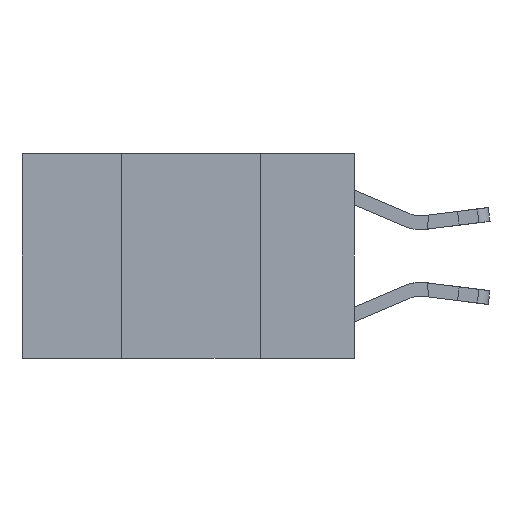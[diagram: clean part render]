
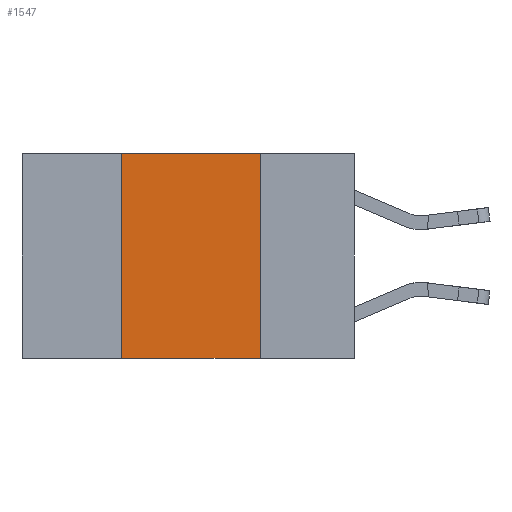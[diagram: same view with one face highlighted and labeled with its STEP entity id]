
A CAD part, left-side view. The second image highlights one B-rep face of the part: STEP entity #1547.
In plain terms, the highlighted planar face has unit normal (-1, 0, 0).
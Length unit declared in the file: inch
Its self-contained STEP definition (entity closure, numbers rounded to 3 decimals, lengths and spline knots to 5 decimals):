
#706 = VECTOR ( 'NONE', #12250, 39.37008 ) ;
#799 = LINE ( 'NONE', #14704, #10522 ) ;
#994 = DIRECTION ( 'NONE',  ( 0., -1., 0. ) ) ;
#1257 = VERTEX_POINT ( 'NONE', #6900 ) ;
#1547 = ADVANCED_FACE ( 'NONE', ( #10801 ), #2718, .F. ) ;
#2061 = VECTOR ( 'NONE', #11833, 39.37008 ) ;
#2718 = PLANE ( 'NONE',  #9936 ) ;
#3215 = ORIENTED_EDGE ( 'NONE', *, *, #4016, .F. ) ;
#3453 = CARTESIAN_POINT ( 'NONE',  ( 0., 0.6, -0.37 ) ) ;
#3618 = VERTEX_POINT ( 'NONE', #4906 ) ;
#3799 = ORIENTED_EDGE ( 'NONE', *, *, #6471, .F. ) ;
#4015 = LINE ( 'NONE', #11058, #706 ) ;
#4016 = EDGE_CURVE ( 'NONE', #3618, #1257, #8946, .T. ) ;
#4339 = EDGE_LOOP ( 'NONE', ( #10075, #3215, #3799, #9729 ) ) ;
#4906 = CARTESIAN_POINT ( 'NONE',  ( 0., 0.42, 0. ) ) ;
#5204 = DIRECTION ( 'NONE',  ( 0., 0., -1. ) ) ;
#5655 = EDGE_CURVE ( 'NONE', #6476, #13946, #10934, .T. ) ;
#5852 = CARTESIAN_POINT ( 'NONE',  ( 0., 0.6, 0. ) ) ;
#6471 = EDGE_CURVE ( 'NONE', #6476, #3618, #799, .T. ) ;
#6476 = VERTEX_POINT ( 'NONE', #13464 ) ;
#6900 = CARTESIAN_POINT ( 'NONE',  ( 0., 0.17, 0. ) ) ;
#7545 = DIRECTION ( 'NONE',  ( 0., 0., 1. ) ) ;
#7910 = CARTESIAN_POINT ( 'NONE',  ( 0., 0.17, -0.37 ) ) ;
#8946 = LINE ( 'NONE', #5852, #2061 ) ;
#9697 = EDGE_CURVE ( 'NONE', #1257, #13946, #4015, .T. ) ;
#9729 = ORIENTED_EDGE ( 'NONE', *, *, #5655, .T. ) ;
#9936 = AXIS2_PLACEMENT_3D ( 'NONE', #11197, #12388, #5204 ) ;
#10075 = ORIENTED_EDGE ( 'NONE', *, *, #9697, .F. ) ;
#10522 = VECTOR ( 'NONE', #7545, 39.37008 ) ;
#10551 = VECTOR ( 'NONE', #994, 39.37008 ) ;
#10801 = FACE_OUTER_BOUND ( 'NONE', #4339, .T. ) ;
#10934 = LINE ( 'NONE', #3453, #10551 ) ;
#11058 = CARTESIAN_POINT ( 'NONE',  ( 0., 0.17, 0. ) ) ;
#11197 = CARTESIAN_POINT ( 'NONE',  ( 0., 0.6, 0. ) ) ;
#11833 = DIRECTION ( 'NONE',  ( 0., -1., 0. ) ) ;
#12250 = DIRECTION ( 'NONE',  ( 0., 0., -1. ) ) ;
#12388 = DIRECTION ( 'NONE',  ( 1., 0., 0. ) ) ;
#13464 = CARTESIAN_POINT ( 'NONE',  ( 0., 0.42, -0.37 ) ) ;
#13946 = VERTEX_POINT ( 'NONE', #7910 ) ;
#14704 = CARTESIAN_POINT ( 'NONE',  ( 0., 0.42, 0. ) ) ;
